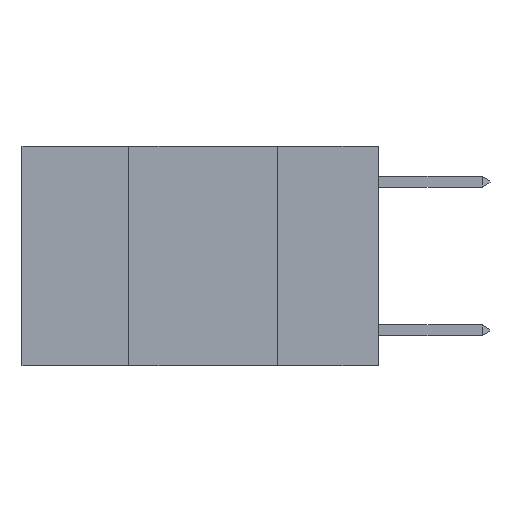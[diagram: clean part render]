
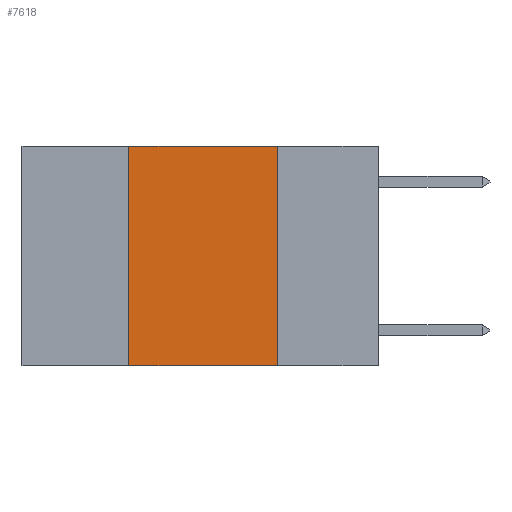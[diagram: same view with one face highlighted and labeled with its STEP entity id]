
A CAD part, left-side view. The second image highlights one B-rep face of the part: STEP entity #7618.
In plain terms, the highlighted planar face has unit normal (-1, 0, 0).
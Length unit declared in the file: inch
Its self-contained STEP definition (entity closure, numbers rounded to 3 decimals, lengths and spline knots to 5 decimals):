
#5 = VECTOR ( 'NONE', #2976, 39.37008 ) ;
#112 = CARTESIAN_POINT ( 'NONE',  ( 0., 0.42, 0. ) ) ;
#547 = LINE ( 'NONE', #7382, #3932 ) ;
#864 = LINE ( 'NONE', #112, #6137 ) ;
#917 = DIRECTION ( 'NONE',  ( 0., 0., 1. ) ) ;
#991 = LINE ( 'NONE', #3498, #3739 ) ;
#1151 = VERTEX_POINT ( 'NONE', #1485 ) ;
#1378 = EDGE_CURVE ( 'NONE', #3276, #9555, #991, .T. ) ;
#1485 = CARTESIAN_POINT ( 'NONE',  ( 0., 0.42, 0. ) ) ;
#2564 = DIRECTION ( 'NONE',  ( 1., 0., 0. ) ) ;
#2698 = EDGE_CURVE ( 'NONE', #1151, #3276, #547, .T. ) ;
#2854 = VERTEX_POINT ( 'NONE', #9609 ) ;
#2976 = DIRECTION ( 'NONE',  ( 0., -1., 0. ) ) ;
#3034 = CARTESIAN_POINT ( 'NONE',  ( 0., 0.17, -0.37 ) ) ;
#3276 = VERTEX_POINT ( 'NONE', #3928 ) ;
#3396 = AXIS2_PLACEMENT_3D ( 'NONE', #8544, #2564, #4823 ) ;
#3498 = CARTESIAN_POINT ( 'NONE',  ( 0., 0.17, 0. ) ) ;
#3739 = VECTOR ( 'NONE', #8683, 39.37008 ) ;
#3837 = EDGE_CURVE ( 'NONE', #2854, #9555, #8190, .T. ) ;
#3918 = EDGE_CURVE ( 'NONE', #2854, #1151, #864, .T. ) ;
#3928 = CARTESIAN_POINT ( 'NONE',  ( 0., 0.17, 0. ) ) ;
#3932 = VECTOR ( 'NONE', #8829, 39.37008 ) ;
#4032 = EDGE_LOOP ( 'NONE', ( #5013, #5514, #6197, #6825 ) ) ;
#4823 = DIRECTION ( 'NONE',  ( 0., 0., -1. ) ) ;
#5013 = ORIENTED_EDGE ( 'NONE', *, *, #1378, .F. ) ;
#5514 = ORIENTED_EDGE ( 'NONE', *, *, #2698, .F. ) ;
#6137 = VECTOR ( 'NONE', #917, 39.37008 ) ;
#6197 = ORIENTED_EDGE ( 'NONE', *, *, #3918, .F. ) ;
#6825 = ORIENTED_EDGE ( 'NONE', *, *, #3837, .T. ) ;
#7042 = FACE_OUTER_BOUND ( 'NONE', #4032, .T. ) ;
#7362 = CARTESIAN_POINT ( 'NONE',  ( 0., 0.6, -0.37 ) ) ;
#7382 = CARTESIAN_POINT ( 'NONE',  ( 0., 0.6, 0. ) ) ;
#7618 = ADVANCED_FACE ( 'NONE', ( #7042 ), #9365, .F. ) ;
#8190 = LINE ( 'NONE', #7362, #5 ) ;
#8544 = CARTESIAN_POINT ( 'NONE',  ( 0., 0.6, 0. ) ) ;
#8683 = DIRECTION ( 'NONE',  ( 0., 0., -1. ) ) ;
#8829 = DIRECTION ( 'NONE',  ( 0., -1., 0. ) ) ;
#9365 = PLANE ( 'NONE',  #3396 ) ;
#9555 = VERTEX_POINT ( 'NONE', #3034 ) ;
#9609 = CARTESIAN_POINT ( 'NONE',  ( 0., 0.42, -0.37 ) ) ;
